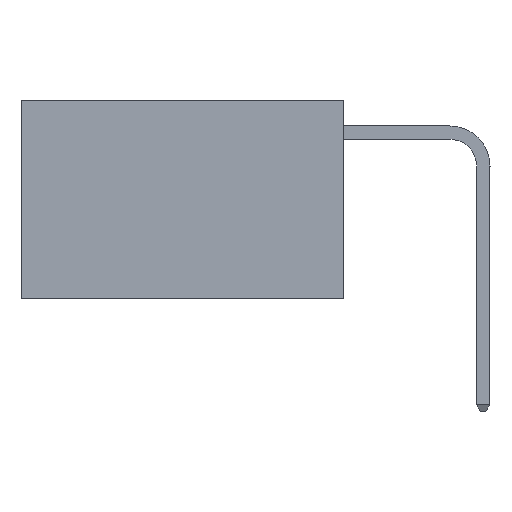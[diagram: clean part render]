
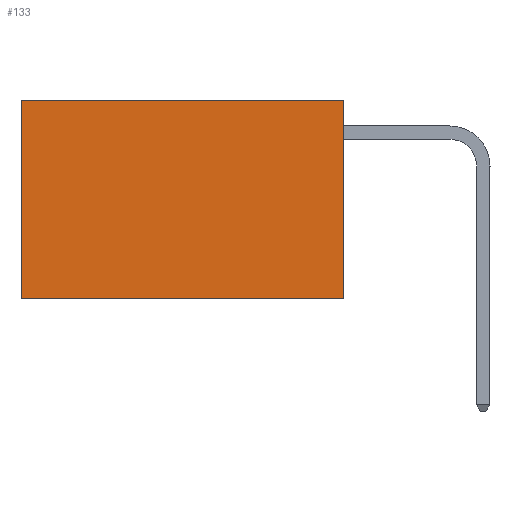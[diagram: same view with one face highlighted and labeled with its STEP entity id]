
A CAD part, left-side view. The second image highlights one B-rep face of the part: STEP entity #133.
In plain terms, the highlighted planar face has unit normal (-1, 0, 0).
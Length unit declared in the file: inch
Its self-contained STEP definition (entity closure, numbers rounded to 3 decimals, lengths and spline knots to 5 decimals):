
#133 = ADVANCED_FACE ( 'NONE', ( #9934 ), #2454, .F. ) ;
#214 = LINE ( 'NONE', #255, #8002 ) ;
#255 = CARTESIAN_POINT ( 'NONE',  ( 0.2625, 0., 0. ) ) ;
#294 = ORIENTED_EDGE ( 'NONE', *, *, #7352, .T. ) ;
#483 = VERTEX_POINT ( 'NONE', #1051 ) ;
#698 = ORIENTED_EDGE ( 'NONE', *, *, #12172, .T. ) ;
#1051 = CARTESIAN_POINT ( 'NONE',  ( 0.2625, 0.6, 0. ) ) ;
#1195 = VECTOR ( 'NONE', #3593, 39.37008 ) ;
#2302 = DIRECTION ( 'NONE',  ( 0., 0., -1. ) ) ;
#2454 = PLANE ( 'NONE',  #10675 ) ;
#2456 = DIRECTION ( 'NONE',  ( 0., 0., -1. ) ) ;
#2587 = CARTESIAN_POINT ( 'NONE',  ( 0.2625, 0., 0. ) ) ;
#3593 = DIRECTION ( 'NONE',  ( 0., 1., 0. ) ) ;
#3896 = CARTESIAN_POINT ( 'NONE',  ( 0.2625, 0.6, 0. ) ) ;
#3946 = EDGE_LOOP ( 'NONE', ( #294, #5773, #8355, #698 ) ) ;
#4601 = EDGE_CURVE ( 'NONE', #7331, #10939, #214, .T. ) ;
#4911 = DIRECTION ( 'NONE',  ( 0., 0., -1. ) ) ;
#5246 = CARTESIAN_POINT ( 'NONE',  ( 0.2625, 0.6, -0.37 ) ) ;
#5404 = VECTOR ( 'NONE', #4911, 39.37008 ) ;
#5609 = DIRECTION ( 'NONE',  ( 1., 0., 0. ) ) ;
#5773 = ORIENTED_EDGE ( 'NONE', *, *, #7393, .F. ) ;
#6909 = CARTESIAN_POINT ( 'NONE',  ( 0.2625, 0., -0.37 ) ) ;
#7331 = VERTEX_POINT ( 'NONE', #12387 ) ;
#7352 = EDGE_CURVE ( 'NONE', #483, #7640, #10466, .T. ) ;
#7393 = EDGE_CURVE ( 'NONE', #10939, #7640, #12636, .T. ) ;
#7640 = VERTEX_POINT ( 'NONE', #5246 ) ;
#8002 = VECTOR ( 'NONE', #2456, 39.37008 ) ;
#8236 = CARTESIAN_POINT ( 'NONE',  ( 0.2625, 0., 0. ) ) ;
#8355 = ORIENTED_EDGE ( 'NONE', *, *, #4601, .F. ) ;
#9050 = LINE ( 'NONE', #2587, #1195 ) ;
#9716 = CARTESIAN_POINT ( 'NONE',  ( 0.2625, 0., -0.37 ) ) ;
#9934 = FACE_OUTER_BOUND ( 'NONE', #3946, .T. ) ;
#10466 = LINE ( 'NONE', #3896, #5404 ) ;
#10675 = AXIS2_PLACEMENT_3D ( 'NONE', #8236, #5609, #2302 ) ;
#10763 = VECTOR ( 'NONE', #12511, 39.37008 ) ;
#10939 = VERTEX_POINT ( 'NONE', #9716 ) ;
#12172 = EDGE_CURVE ( 'NONE', #7331, #483, #9050, .T. ) ;
#12387 = CARTESIAN_POINT ( 'NONE',  ( 0.2625, 0., 0. ) ) ;
#12511 = DIRECTION ( 'NONE',  ( 0., 1., 0. ) ) ;
#12636 = LINE ( 'NONE', #6909, #10763 ) ;
